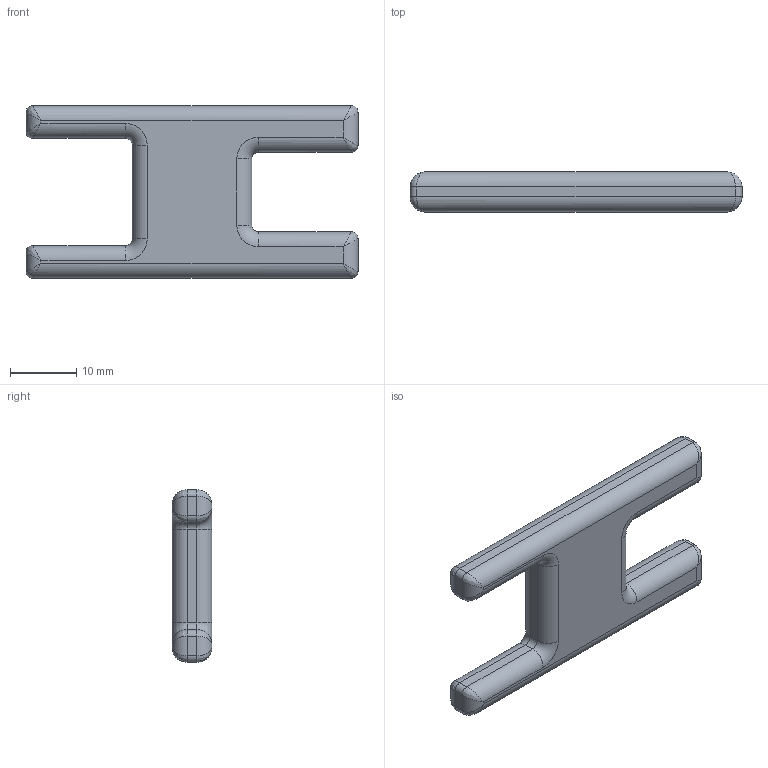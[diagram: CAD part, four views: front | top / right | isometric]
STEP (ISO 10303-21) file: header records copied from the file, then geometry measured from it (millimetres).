
FILE_DESCRIPTION(/* description */ (''),/* implementation_level */ '2;1');
FILE_NAME(/* name */ '//hi-power_3rd-hand v6.step',/* time_stamp */ '2022-05-12T19:39:33-07:00',/* author */ ('freeman1337'),/* organization */ (''),/* preprocessor_version */ 'ST-DEVELOPER v18.1',/* originating_system */ 'Autodesk Translation Framework v10.14.0.1471',/* authorisation */ '');
FILE_SCHEMA (('AUTOMOTIVE_DESIGN { 1 0 10303 214 3 1 1 }'));
Length unit declared in the file: millimetre
Products named in the file (1): hi-power_3rd-hand
Bounding box: 50 x 6 x 26 mm (x, y, z)
Volume: 4615.5 mm3; surface area: 2627.2 mm2
Topology: 1 solids, 1 shells, 220 faces, 573 edges, 350 vertices
Faces by surface type: bspline 105, plane 71, cylinder 36, torus 8
Entity records: 7797 total; most frequent: CARTESIAN_POINT 3105, ORIENTED_EDGE 1114, DIRECTION 691, EDGE_CURVE 557, VERTEX_POINT 350, LINE 299, VECTOR 299, EDGE_LOOP 231
